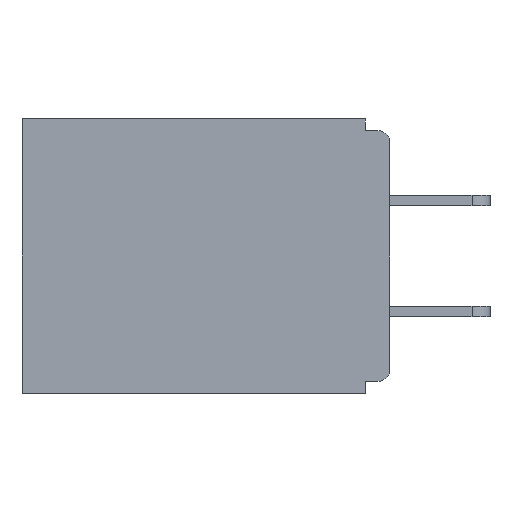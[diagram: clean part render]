
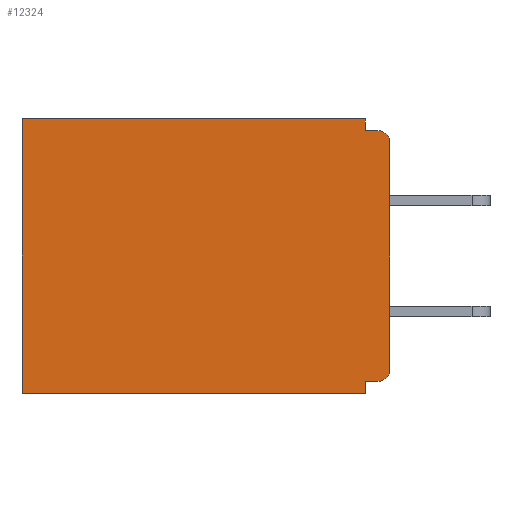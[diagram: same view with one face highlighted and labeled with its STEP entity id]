
A CAD part, left-side view. The second image highlights one B-rep face of the part: STEP entity #12324.
In plain terms, the highlighted planar face has unit normal (-1, 0, 0).
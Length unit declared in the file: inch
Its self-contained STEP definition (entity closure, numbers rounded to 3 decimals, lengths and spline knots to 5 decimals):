
#29 = PLANE ( 'NONE',  #11681 ) ;
#66 = DIRECTION ( 'NONE',  ( 1., 0., 0. ) ) ;
#68 = CARTESIAN_POINT ( 'NONE',  ( 0.298, 0.031, -0.343 ) ) ;
#145 = CARTESIAN_POINT ( 'NONE',  ( 0.298, 0.46, -0.343 ) ) ;
#159 = DIRECTION ( 'NONE',  ( 0., 1., 0. ) ) ;
#615 = DIRECTION ( 'NONE',  ( 0., 1., 0. ) ) ;
#639 = ORIENTED_EDGE ( 'NONE', *, *, #12047, .T. ) ;
#1119 = DIRECTION ( 'NONE',  ( 0., 0., -1. ) ) ;
#1329 = VECTOR ( 'NONE', #12394, 39.37008 ) ;
#1484 = ORIENTED_EDGE ( 'NONE', *, *, #6526, .T. ) ;
#1676 = ORIENTED_EDGE ( 'NONE', *, *, #8935, .F. ) ;
#2142 = CARTESIAN_POINT ( 'NONE',  ( 0.298, 0.015, -0.03 ) ) ;
#2189 = DIRECTION ( 'NONE',  ( 0., 0., -1. ) ) ;
#2352 = VECTOR ( 'NONE', #7719, 39.37008 ) ;
#2369 = CARTESIAN_POINT ( 'NONE',  ( 0.298, 0., -0.015 ) ) ;
#2474 = EDGE_CURVE ( 'NONE', #3675, #13163, #9739, .T. ) ;
#2577 = DIRECTION ( 'NONE',  ( 0., 0., -1. ) ) ;
#2672 = ORIENTED_EDGE ( 'NONE', *, *, #12371, .T. ) ;
#2784 = CIRCLE ( 'NONE', #11582, 0.015 ) ;
#2836 = LINE ( 'NONE', #7993, #4946 ) ;
#2860 = CARTESIAN_POINT ( 'NONE',  ( 0.298, 0.031, -0.328 ) ) ;
#3265 = CARTESIAN_POINT ( 'NONE',  ( 0.298, 0., 0. ) ) ;
#3440 = LINE ( 'NONE', #11576, #5566 ) ;
#3675 = VERTEX_POINT ( 'NONE', #11946 ) ;
#4120 = CARTESIAN_POINT ( 'NONE',  ( 0.298, 0., -0.328 ) ) ;
#4243 = VECTOR ( 'NONE', #2577, 39.37008 ) ;
#4261 = CARTESIAN_POINT ( 'NONE',  ( 0.298, 0.031, -0.343 ) ) ;
#4361 = CARTESIAN_POINT ( 'NONE',  ( 0.298, 0.015, -0.328 ) ) ;
#4556 = LINE ( 'NONE', #6808, #4243 ) ;
#4773 = DIRECTION ( 'NONE',  ( 0., 0., -1. ) ) ;
#4826 = DIRECTION ( 'NONE',  ( 0., 0., -1. ) ) ;
#4940 = CARTESIAN_POINT ( 'NONE',  ( 0.298, 0.015, -0.015 ) ) ;
#4946 = VECTOR ( 'NONE', #4826, 39.37008 ) ;
#5226 = CARTESIAN_POINT ( 'NONE',  ( 0.298, 0., 0. ) ) ;
#5306 = DIRECTION ( 'NONE',  ( 0., 0., -1. ) ) ;
#5448 = CARTESIAN_POINT ( 'NONE',  ( 0.298, 0.015, -0.313 ) ) ;
#5566 = VECTOR ( 'NONE', #2189, 39.37008 ) ;
#5893 = EDGE_CURVE ( 'NONE', #6420, #8594, #13112, .T. ) ;
#5983 = AXIS2_PLACEMENT_3D ( 'NONE', #2142, #8500, #9394 ) ;
#5986 = ORIENTED_EDGE ( 'NONE', *, *, #10539, .F. ) ;
#6258 = VERTEX_POINT ( 'NONE', #4940 ) ;
#6420 = VERTEX_POINT ( 'NONE', #4361 ) ;
#6526 = EDGE_CURVE ( 'NONE', #11306, #6258, #8772, .T. ) ;
#6683 = LINE ( 'NONE', #11997, #6699 ) ;
#6699 = VECTOR ( 'NONE', #615, 39.37008 ) ;
#6724 = CARTESIAN_POINT ( 'NONE',  ( 0.298, 0., -0.03 ) ) ;
#6808 = CARTESIAN_POINT ( 'NONE',  ( 0.298, 0.031, -0.343 ) ) ;
#6858 = VECTOR ( 'NONE', #5306, 39.37008 ) ;
#7270 = VERTEX_POINT ( 'NONE', #8901 ) ;
#7719 = DIRECTION ( 'NONE',  ( 0., -1., 0. ) ) ;
#7993 = CARTESIAN_POINT ( 'NONE',  ( 0.298, 0., 0. ) ) ;
#8253 = VERTEX_POINT ( 'NONE', #68 ) ;
#8443 = VERTEX_POINT ( 'NONE', #9537 ) ;
#8500 = DIRECTION ( 'NONE',  ( -1., 0., 0. ) ) ;
#8594 = VERTEX_POINT ( 'NONE', #2860 ) ;
#8772 = CIRCLE ( 'NONE', #5983, 0.015 ) ;
#8887 = VERTEX_POINT ( 'NONE', #145 ) ;
#8901 = CARTESIAN_POINT ( 'NONE',  ( 0.298, 0.46, 0. ) ) ;
#8935 = EDGE_CURVE ( 'NONE', #13163, #6258, #10141, .T. ) ;
#9089 = EDGE_CURVE ( 'NONE', #11306, #8443, #2836, .T. ) ;
#9377 = ORIENTED_EDGE ( 'NONE', *, *, #9851, .T. ) ;
#9394 = DIRECTION ( 'NONE',  ( 0., 0., -1. ) ) ;
#9537 = CARTESIAN_POINT ( 'NONE',  ( 0.298, 0., -0.313 ) ) ;
#9739 = LINE ( 'NONE', #4261, #6858 ) ;
#9851 = EDGE_CURVE ( 'NONE', #7270, #8887, #3440, .T. ) ;
#10141 = LINE ( 'NONE', #2369, #2352 ) ;
#10388 = FACE_OUTER_BOUND ( 'NONE', #13372, .T. ) ;
#10489 = ORIENTED_EDGE ( 'NONE', *, *, #5893, .F. ) ;
#10539 = EDGE_CURVE ( 'NONE', #8594, #8253, #4556, .T. ) ;
#10610 = ORIENTED_EDGE ( 'NONE', *, *, #2474, .F. ) ;
#10616 = DIRECTION ( 'NONE',  ( -1., 0., 0. ) ) ;
#11154 = EDGE_CURVE ( 'NONE', #8253, #8887, #6683, .T. ) ;
#11209 = VECTOR ( 'NONE', #159, 39.37008 ) ;
#11306 = VERTEX_POINT ( 'NONE', #6724 ) ;
#11576 = CARTESIAN_POINT ( 'NONE',  ( 0.298, 0.46, 0. ) ) ;
#11582 = AXIS2_PLACEMENT_3D ( 'NONE', #5448, #10616, #4773 ) ;
#11599 = ORIENTED_EDGE ( 'NONE', *, *, #9089, .F. ) ;
#11681 = AXIS2_PLACEMENT_3D ( 'NONE', #5226, #66, #1119 ) ;
#11838 = LINE ( 'NONE', #3265, #11209 ) ;
#11946 = CARTESIAN_POINT ( 'NONE',  ( 0.298, 0.031, 0. ) ) ;
#11997 = CARTESIAN_POINT ( 'NONE',  ( 0.298, 0., -0.343 ) ) ;
#12047 = EDGE_CURVE ( 'NONE', #6420, #8443, #2784, .T. ) ;
#12324 = ADVANCED_FACE ( 'NONE', ( #10388 ), #29, .F. ) ;
#12371 = EDGE_CURVE ( 'NONE', #3675, #7270, #11838, .T. ) ;
#12394 = DIRECTION ( 'NONE',  ( 0., 1., 0. ) ) ;
#12642 = CARTESIAN_POINT ( 'NONE',  ( 0.298, 0.031, -0.015 ) ) ;
#13112 = LINE ( 'NONE', #4120, #1329 ) ;
#13114 = ORIENTED_EDGE ( 'NONE', *, *, #11154, .F. ) ;
#13163 = VERTEX_POINT ( 'NONE', #12642 ) ;
#13372 = EDGE_LOOP ( 'NONE', ( #1484, #1676, #10610, #2672, #9377, #13114, #5986, #10489, #639, #11599 ) ) ;
